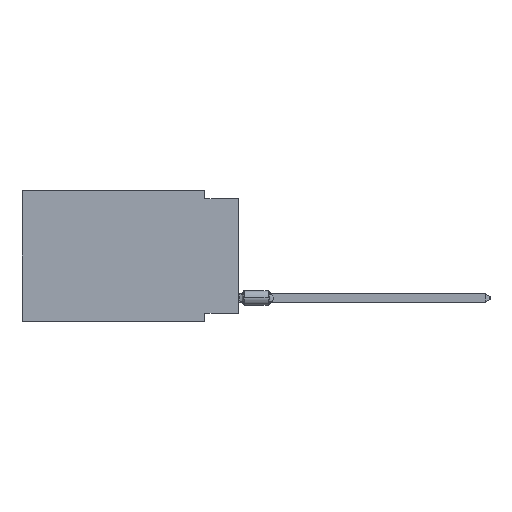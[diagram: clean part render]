
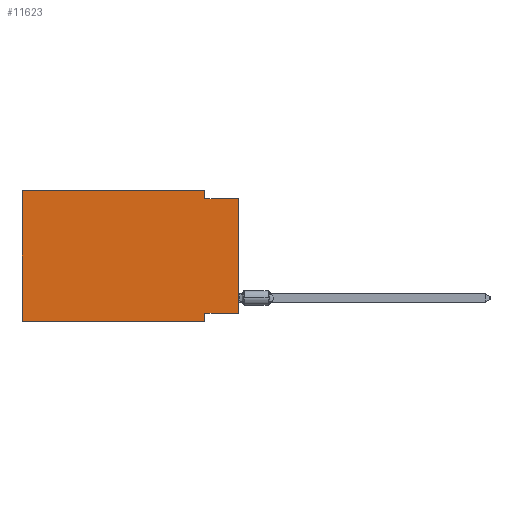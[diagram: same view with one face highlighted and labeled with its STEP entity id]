
A CAD part, left-side view. The second image highlights one B-rep face of the part: STEP entity #11623.
In plain terms, the highlighted planar face has unit normal (-1, 0, 0).
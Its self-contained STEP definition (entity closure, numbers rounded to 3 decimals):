
#196 = LINE ( 'NONE', #9641, #23398 ) ;
#2127 = CARTESIAN_POINT ( 'NONE',  ( 0., 16.383, -9.906 ) ) ;
#2534 = AXIS2_PLACEMENT_3D ( 'NONE', #25909, #6775, #35961 ) ;
#3231 = CARTESIAN_POINT ( 'NONE',  ( 0., 16.383, 0. ) ) ;
#4913 = CARTESIAN_POINT ( 'NONE',  ( 0., 0., -9.271 ) ) ;
#5623 = ORIENTED_EDGE ( 'NONE', *, *, #33802, .F. ) ;
#6775 = DIRECTION ( 'NONE',  ( 1., 0., 0. ) ) ;
#7734 = VECTOR ( 'NONE', #40013, 1000. ) ;
#7857 = VERTEX_POINT ( 'NONE', #41164 ) ;
#8591 = VECTOR ( 'NONE', #21163, 1000. ) ;
#9641 = CARTESIAN_POINT ( 'NONE',  ( 0., 0., -0.635 ) ) ;
#10622 = ORIENTED_EDGE ( 'NONE', *, *, #33572, .F. ) ;
#11623 = ADVANCED_FACE ( 'NONE', ( #12691 ), #25511, .F. ) ;
#11781 = VECTOR ( 'NONE', #35309, 1000. ) ;
#12201 = CARTESIAN_POINT ( 'NONE',  ( 0., 0., -9.271 ) ) ;
#12691 = FACE_OUTER_BOUND ( 'NONE', #36283, .T. ) ;
#13012 = DIRECTION ( 'NONE',  ( 0., -1., 0. ) ) ;
#13712 = CARTESIAN_POINT ( 'NONE',  ( 0., 2.54, -9.906 ) ) ;
#14148 = VERTEX_POINT ( 'NONE', #13712 ) ;
#14412 = ORIENTED_EDGE ( 'NONE', *, *, #36824, .F. ) ;
#14596 = LINE ( 'NONE', #27406, #7734 ) ;
#14607 = LINE ( 'NONE', #4913, #23032 ) ;
#14887 = EDGE_CURVE ( 'NONE', #21823, #22421, #196, .T. ) ;
#15532 = VERTEX_POINT ( 'NONE', #2127 ) ;
#16072 = DIRECTION ( 'NONE',  ( 0., 0., 1. ) ) ;
#16406 = LINE ( 'NONE', #34687, #11781 ) ;
#18570 = DIRECTION ( 'NONE',  ( 0., 0., 1. ) ) ;
#18792 = CARTESIAN_POINT ( 'NONE',  ( 0., 0., 0. ) ) ;
#21163 = DIRECTION ( 'NONE',  ( 0., -1., 0. ) ) ;
#21823 = VERTEX_POINT ( 'NONE', #29674 ) ;
#22017 = ORIENTED_EDGE ( 'NONE', *, *, #36679, .F. ) ;
#22263 = CARTESIAN_POINT ( 'NONE',  ( 0., 0., -0.635 ) ) ;
#22291 = CARTESIAN_POINT ( 'NONE',  ( 0., 2.54, -9.271 ) ) ;
#22369 = LINE ( 'NONE', #3231, #27723 ) ;
#22421 = VERTEX_POINT ( 'NONE', #22263 ) ;
#23032 = VECTOR ( 'NONE', #27614, 1000. ) ;
#23398 = VECTOR ( 'NONE', #13012, 1000. ) ;
#24089 = ORIENTED_EDGE ( 'NONE', *, *, #28638, .T. ) ;
#24335 = ORIENTED_EDGE ( 'NONE', *, *, #40546, .F. ) ;
#25511 = PLANE ( 'NONE',  #2534 ) ;
#25909 = CARTESIAN_POINT ( 'NONE',  ( 0., 16.383, 0. ) ) ;
#26467 = VECTOR ( 'NONE', #18570, 1000. ) ;
#27241 = VECTOR ( 'NONE', #34548, 1000. ) ;
#27406 = CARTESIAN_POINT ( 'NONE',  ( 0., 2.54, -9.906 ) ) ;
#27614 = DIRECTION ( 'NONE',  ( 0., 1., 0. ) ) ;
#27723 = VECTOR ( 'NONE', #16072, 1000. ) ;
#28638 = EDGE_CURVE ( 'NONE', #38097, #22421, #37678, .T. ) ;
#28902 = ORIENTED_EDGE ( 'NONE', *, *, #38205, .T. ) ;
#29674 = CARTESIAN_POINT ( 'NONE',  ( 0., 2.54, -0.635 ) ) ;
#29986 = VERTEX_POINT ( 'NONE', #40193 ) ;
#30549 = VERTEX_POINT ( 'NONE', #22291 ) ;
#33572 = EDGE_CURVE ( 'NONE', #38097, #30549, #14607, .T. ) ;
#33802 = EDGE_CURVE ( 'NONE', #15532, #29986, #22369, .T. ) ;
#34548 = DIRECTION ( 'NONE',  ( 0., 0., -1. ) ) ;
#34614 = CARTESIAN_POINT ( 'NONE',  ( 0., 16.383, 0. ) ) ;
#34687 = CARTESIAN_POINT ( 'NONE',  ( 0., 16.383, -9.906 ) ) ;
#35174 = CARTESIAN_POINT ( 'NONE',  ( 0., 2.54, 0. ) ) ;
#35309 = DIRECTION ( 'NONE',  ( 0., -1., 0. ) ) ;
#35961 = DIRECTION ( 'NONE',  ( 0., 0., -1. ) ) ;
#36283 = EDGE_LOOP ( 'NONE', ( #24089, #39892, #14412, #24335, #5623, #28902, #22017, #10622 ) ) ;
#36679 = EDGE_CURVE ( 'NONE', #30549, #14148, #14596, .T. ) ;
#36824 = EDGE_CURVE ( 'NONE', #7857, #21823, #37900, .T. ) ;
#37319 = LINE ( 'NONE', #34614, #8591 ) ;
#37678 = LINE ( 'NONE', #18792, #26467 ) ;
#37900 = LINE ( 'NONE', #35174, #27241 ) ;
#38097 = VERTEX_POINT ( 'NONE', #12201 ) ;
#38205 = EDGE_CURVE ( 'NONE', #15532, #14148, #16406, .T. ) ;
#39892 = ORIENTED_EDGE ( 'NONE', *, *, #14887, .F. ) ;
#40013 = DIRECTION ( 'NONE',  ( 0., 0., -1. ) ) ;
#40193 = CARTESIAN_POINT ( 'NONE',  ( 0., 16.383, 0. ) ) ;
#40546 = EDGE_CURVE ( 'NONE', #29986, #7857, #37319, .T. ) ;
#41164 = CARTESIAN_POINT ( 'NONE',  ( 0., 2.54, 0. ) ) ;
